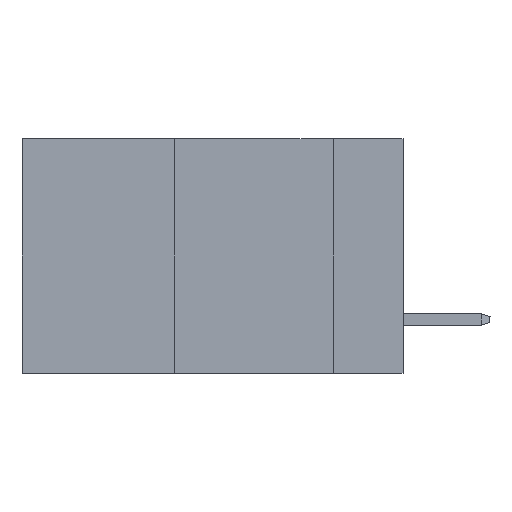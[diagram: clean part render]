
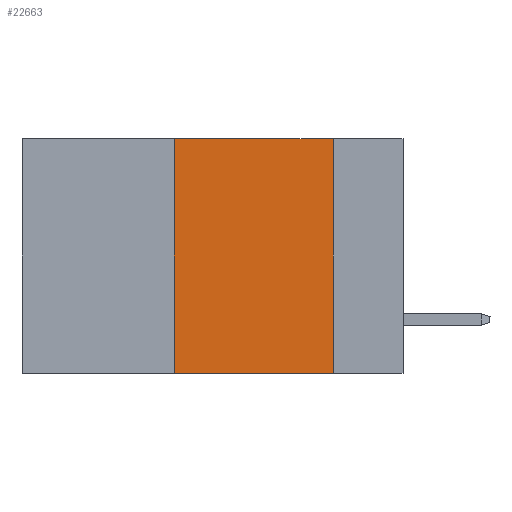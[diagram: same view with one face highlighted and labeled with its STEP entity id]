
A CAD part, left-side view. The second image highlights one B-rep face of the part: STEP entity #22663.
In plain terms, the highlighted planar face has unit normal (-1, 0, 0).
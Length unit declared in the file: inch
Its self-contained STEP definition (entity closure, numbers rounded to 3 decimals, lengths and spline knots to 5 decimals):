
#105 = DIRECTION ( 'NONE',  ( 1., 0., 0. ) ) ;
#1220 = DIRECTION ( 'NONE',  ( 0., -1., 0. ) ) ;
#2656 = ORIENTED_EDGE ( 'NONE', *, *, #6385, .T. ) ;
#3100 = EDGE_LOOP ( 'NONE', ( #15418, #10259, #9346, #2656 ) ) ;
#3446 = VECTOR ( 'NONE', #1220, 39.37008 ) ;
#3459 = EDGE_CURVE ( 'NONE', #5966, #23754, #19100, .T. ) ;
#3824 = FACE_OUTER_BOUND ( 'NONE', #3100, .T. ) ;
#4059 = CARTESIAN_POINT ( 'NONE',  ( 0., 0.36, -0.37 ) ) ;
#4732 = DIRECTION ( 'NONE',  ( 0., -1., 0. ) ) ;
#5778 = CARTESIAN_POINT ( 'NONE',  ( 0., 0.36, 0. ) ) ;
#5808 = EDGE_CURVE ( 'NONE', #18817, #12366, #9561, .T. ) ;
#5966 = VERTEX_POINT ( 'NONE', #8587 ) ;
#6272 = CARTESIAN_POINT ( 'NONE',  ( 0., 0.11, 0. ) ) ;
#6385 = EDGE_CURVE ( 'NONE', #18817, #23754, #17809, .T. ) ;
#7417 = DIRECTION ( 'NONE',  ( 0., 0., -1. ) ) ;
#8587 = CARTESIAN_POINT ( 'NONE',  ( 0., 0.11, 0. ) ) ;
#9220 = PLANE ( 'NONE',  #16211 ) ;
#9346 = ORIENTED_EDGE ( 'NONE', *, *, #5808, .F. ) ;
#9561 = LINE ( 'NONE', #11844, #22164 ) ;
#10259 = ORIENTED_EDGE ( 'NONE', *, *, #20020, .F. ) ;
#11586 = VECTOR ( 'NONE', #13847, 39.37008 ) ;
#11844 = CARTESIAN_POINT ( 'NONE',  ( 0., 0.36, 0. ) ) ;
#12267 = CARTESIAN_POINT ( 'NONE',  ( 0., 0.6, 0. ) ) ;
#12366 = VERTEX_POINT ( 'NONE', #5778 ) ;
#12388 = LINE ( 'NONE', #12267, #3446 ) ;
#13847 = DIRECTION ( 'NONE',  ( 0., 0., -1. ) ) ;
#14221 = CARTESIAN_POINT ( 'NONE',  ( 0., 0.6, -0.37 ) ) ;
#15418 = ORIENTED_EDGE ( 'NONE', *, *, #3459, .F. ) ;
#16211 = AXIS2_PLACEMENT_3D ( 'NONE', #20253, #105, #7417 ) ;
#17809 = LINE ( 'NONE', #14221, #17990 ) ;
#17990 = VECTOR ( 'NONE', #4732, 39.37008 ) ;
#18239 = CARTESIAN_POINT ( 'NONE',  ( 0., 0.11, -0.37 ) ) ;
#18817 = VERTEX_POINT ( 'NONE', #4059 ) ;
#19033 = DIRECTION ( 'NONE',  ( 0., 0., 1. ) ) ;
#19100 = LINE ( 'NONE', #6272, #11586 ) ;
#20020 = EDGE_CURVE ( 'NONE', #12366, #5966, #12388, .T. ) ;
#20253 = CARTESIAN_POINT ( 'NONE',  ( 0., 0.6, 0. ) ) ;
#22164 = VECTOR ( 'NONE', #19033, 39.37008 ) ;
#22663 = ADVANCED_FACE ( 'NONE', ( #3824 ), #9220, .F. ) ;
#23754 = VERTEX_POINT ( 'NONE', #18239 ) ;
